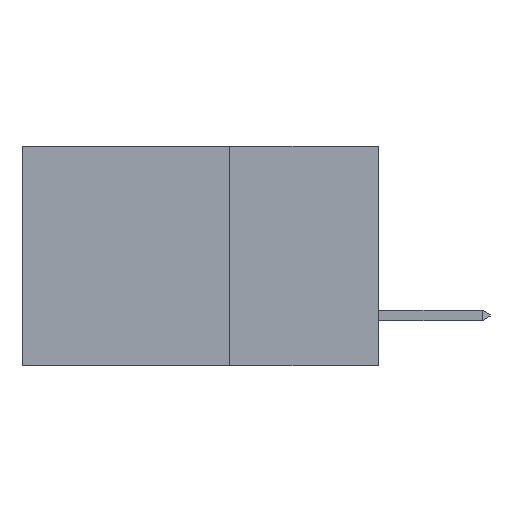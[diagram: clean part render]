
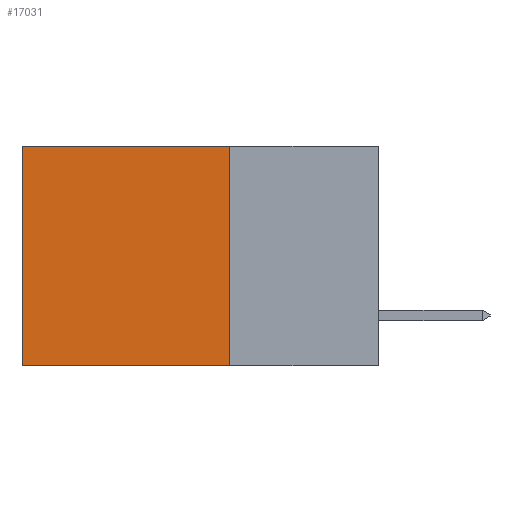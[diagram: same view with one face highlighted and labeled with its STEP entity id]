
A CAD part, left-side view. The second image highlights one B-rep face of the part: STEP entity #17031.
In plain terms, the highlighted planar face has unit normal (-1, 0, 0).
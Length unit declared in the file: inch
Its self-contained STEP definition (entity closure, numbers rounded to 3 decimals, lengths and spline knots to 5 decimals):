
#409 = CARTESIAN_POINT ( 'NONE',  ( 0.298, 0.25, 0. ) ) ;
#1808 = LINE ( 'NONE', #3996, #5184 ) ;
#1871 = CARTESIAN_POINT ( 'NONE',  ( 0.298, 0.25, 0. ) ) ;
#1938 = PLANE ( 'NONE',  #14896 ) ;
#2568 = DIRECTION ( 'NONE',  ( 0., 1., 0. ) ) ;
#3627 = DIRECTION ( 'NONE',  ( 0., 0., -1. ) ) ;
#3996 = CARTESIAN_POINT ( 'NONE',  ( 0.298, 0.25, 0. ) ) ;
#4132 = VECTOR ( 'NONE', #11819, 39.37008 ) ;
#4880 = VERTEX_POINT ( 'NONE', #15066 ) ;
#5184 = VECTOR ( 'NONE', #5671, 39.37008 ) ;
#5366 = DIRECTION ( 'NONE',  ( 0., 0., -1. ) ) ;
#5671 = DIRECTION ( 'NONE',  ( 0., 1., 0. ) ) ;
#6027 = LINE ( 'NONE', #10348, #13862 ) ;
#6951 = ORIENTED_EDGE ( 'NONE', *, *, #13531, .F. ) ;
#7546 = ORIENTED_EDGE ( 'NONE', *, *, #20961, .F. ) ;
#7572 = ORIENTED_EDGE ( 'NONE', *, *, #18420, .T. ) ;
#7674 = VECTOR ( 'NONE', #2568, 39.37008 ) ;
#8486 = LINE ( 'NONE', #10107, #4132 ) ;
#9127 = CARTESIAN_POINT ( 'NONE',  ( 0.298, 0.25, -0.37 ) ) ;
#9600 = CARTESIAN_POINT ( 'NONE',  ( 0.298, 0.25, -0.37 ) ) ;
#10107 = CARTESIAN_POINT ( 'NONE',  ( 0.298, 0.25, 0. ) ) ;
#10348 = CARTESIAN_POINT ( 'NONE',  ( 0.298, 0.6, 0. ) ) ;
#11819 = DIRECTION ( 'NONE',  ( 0., 0., -1. ) ) ;
#12065 = EDGE_LOOP ( 'NONE', ( #7572, #6951, #7546, #16522 ) ) ;
#13531 = EDGE_CURVE ( 'NONE', #20793, #4880, #20904, .T. ) ;
#13607 = DIRECTION ( 'NONE',  ( 1., 0., 0. ) ) ;
#13862 = VECTOR ( 'NONE', #5366, 39.37008 ) ;
#14749 = CARTESIAN_POINT ( 'NONE',  ( 0.298, 0.6, 0. ) ) ;
#14896 = AXIS2_PLACEMENT_3D ( 'NONE', #1871, #13607, #3627 ) ;
#15066 = CARTESIAN_POINT ( 'NONE',  ( 0.298, 0.6, -0.37 ) ) ;
#16522 = ORIENTED_EDGE ( 'NONE', *, *, #20503, .T. ) ;
#17031 = ADVANCED_FACE ( 'NONE', ( #17541 ), #1938, .F. ) ;
#17541 = FACE_OUTER_BOUND ( 'NONE', #12065, .T. ) ;
#18172 = VERTEX_POINT ( 'NONE', #14749 ) ;
#18420 = EDGE_CURVE ( 'NONE', #18172, #4880, #6027, .T. ) ;
#19158 = VERTEX_POINT ( 'NONE', #409 ) ;
#20503 = EDGE_CURVE ( 'NONE', #19158, #18172, #1808, .T. ) ;
#20793 = VERTEX_POINT ( 'NONE', #9600 ) ;
#20904 = LINE ( 'NONE', #9127, #7674 ) ;
#20961 = EDGE_CURVE ( 'NONE', #19158, #20793, #8486, .T. ) ;
